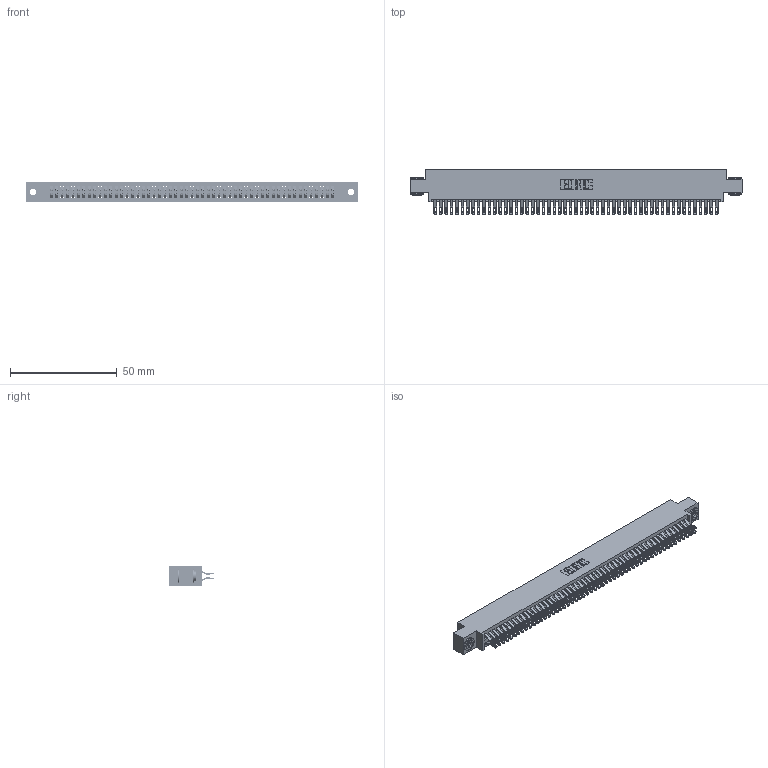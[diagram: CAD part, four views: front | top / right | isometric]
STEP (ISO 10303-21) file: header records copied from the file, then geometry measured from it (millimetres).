
FILE_DESCRIPTION (( 'STEP AP203' ), '1' );
FILE_NAME ('395-106-555-803.STEP', '2018-11-30T17:38:28', ( '' ), ( '' ), 'SwSTEP 2.0', 'SolidWorks 2016', '' );
FILE_SCHEMA (( 'CONFIG_CONTROL_DESIGN' ));
Length unit declared in the file: inch
Products named in the file (4): 345 Part_0.170 Offset - 0.156 Dia-TH; 345-292-001_555 Tail; 345-250-002_345-250-002-102; 395-106-555-803
Assembly tree (109 placements, depth 2):
  395-106-555-803
    345 Part_0.170 Offset - 0.156 Dia-TH
    345-292-001_555 Tail  x106
    345-250-002_345-250-002-102  x2
Bounding box: 155.83 x 21.13 x 9.4 mm (x, y, z)
Volume: 15453 mm3; surface area: 24472.9 mm2
Topology: 109 solids, 109 shells, 6104 faces, 19191 edges, 12790 vertices
Faces by surface type: plane 3380, cylinder 2716, cone 8
Entity records: 41212 total; most frequent: CARTESIAN_POINT 6909, ORIENTED_EDGE 6806, DIRECTION 6077, EDGE_CURVE 3403, VECTOR 3015, LINE 3015, VERTEX_POINT 2266, AXIS2_PLACEMENT_3D 1531
